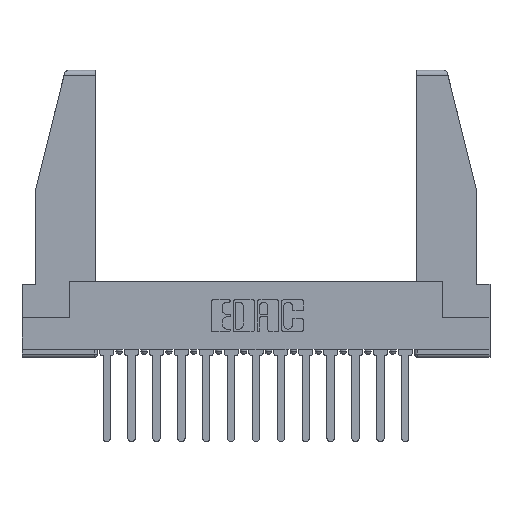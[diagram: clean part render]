
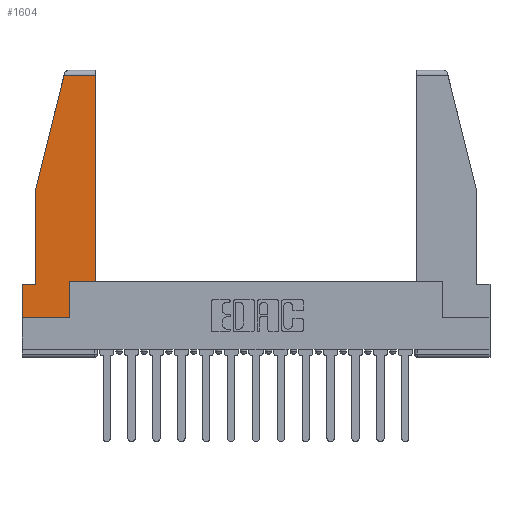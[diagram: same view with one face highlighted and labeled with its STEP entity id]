
A CAD part, top view. The second image highlights one B-rep face of the part: STEP entity #1604.
In plain terms, the highlighted planar face has unit normal (0, 0, 1).
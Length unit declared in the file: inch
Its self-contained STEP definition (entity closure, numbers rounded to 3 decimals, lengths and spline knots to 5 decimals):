
#199 = ORIENTED_EDGE ( 'NONE', *, *, #250, .T. ) ;
#250 = EDGE_CURVE ( 'NONE', #10235, #15832, #759, .T. ) ;
#589 = EDGE_LOOP ( 'NONE', ( #4565, #8580, #4721, #5813, #199, #5199, #11838, #7251, #9016 ) ) ;
#639 = AXIS2_PLACEMENT_3D ( 'NONE', #9587, #5339, #2652 ) ;
#759 = LINE ( 'NONE', #16954, #15724 ) ;
#966 = DIRECTION ( 'NONE',  ( -0.239, -0.971, 0. ) ) ;
#1041 = CARTESIAN_POINT ( 'NONE',  ( 0.461, 1.52, 0. ) ) ;
#1324 = CARTESIAN_POINT ( 'NONE',  ( 0.271, 1.55, 0. ) ) ;
#1604 = ADVANCED_FACE ( 'NONE', ( #13386 ), #8262, .T. ) ;
#1824 = VECTOR ( 'NONE', #15880, 39.37008 ) ;
#1844 = DIRECTION ( 'NONE',  ( 0., -1., 0. ) ) ;
#2352 = CARTESIAN_POINT ( 'NONE',  ( 0.461, 0.223, 0. ) ) ;
#2359 = LINE ( 'NONE', #17128, #13360 ) ;
#2652 = DIRECTION ( 'NONE',  ( 1., 0., 0. ) ) ;
#2764 = CARTESIAN_POINT ( 'NONE',  ( 0.086, 0.8, 0. ) ) ;
#3271 = DIRECTION ( 'NONE',  ( -1., 0., 0. ) ) ;
#3292 = EDGE_CURVE ( 'NONE', #16701, #4306, #10634, .T. ) ;
#3340 = EDGE_CURVE ( 'NONE', #10480, #16760, #6547, .T. ) ;
#3363 = CARTESIAN_POINT ( 'NONE',  ( 0.086, 0.21, 0. ) ) ;
#3607 = EDGE_CURVE ( 'NONE', #9724, #10235, #15353, .T. ) ;
#4048 = LINE ( 'NONE', #9469, #16231 ) ;
#4306 = VERTEX_POINT ( 'NONE', #5192 ) ;
#4406 = CARTESIAN_POINT ( 'NONE',  ( 0., 0.21, 0. ) ) ;
#4565 = ORIENTED_EDGE ( 'NONE', *, *, #11818, .T. ) ;
#4721 = ORIENTED_EDGE ( 'NONE', *, *, #7964, .T. ) ;
#5113 = EDGE_CURVE ( 'NONE', #16760, #8881, #4048, .T. ) ;
#5192 = CARTESIAN_POINT ( 'NONE',  ( 0.2636, 1.52, 0. ) ) ;
#5199 = ORIENTED_EDGE ( 'NONE', *, *, #11905, .T. ) ;
#5339 = DIRECTION ( 'NONE',  ( 0., 0., 1. ) ) ;
#5774 = CARTESIAN_POINT ( 'NONE',  ( 0.086, 0.8, 0. ) ) ;
#5813 = ORIENTED_EDGE ( 'NONE', *, *, #3607, .T. ) ;
#6547 = LINE ( 'NONE', #16063, #16580 ) ;
#6697 = DIRECTION ( 'NONE',  ( 1., 0., 0. ) ) ;
#6747 = VECTOR ( 'NONE', #966, 39.37008 ) ;
#6892 = DIRECTION ( 'NONE',  ( 0., -1., 0. ) ) ;
#7251 = ORIENTED_EDGE ( 'NONE', *, *, #3340, .T. ) ;
#7964 = EDGE_CURVE ( 'NONE', #4306, #9724, #10735, .T. ) ;
#8262 = PLANE ( 'NONE',  #639 ) ;
#8447 = CARTESIAN_POINT ( 'NONE',  ( 0.297, 0.223, 0. ) ) ;
#8580 = ORIENTED_EDGE ( 'NONE', *, *, #3292, .T. ) ;
#8881 = VERTEX_POINT ( 'NONE', #2352 ) ;
#9016 = ORIENTED_EDGE ( 'NONE', *, *, #5113, .T. ) ;
#9469 = CARTESIAN_POINT ( 'NONE',  ( 0.297, 0.223, 0. ) ) ;
#9559 = DIRECTION ( 'NONE',  ( 1., 0., 0. ) ) ;
#9587 = CARTESIAN_POINT ( 'NONE',  ( 0., 0., 0. ) ) ;
#9724 = VERTEX_POINT ( 'NONE', #2764 ) ;
#10235 = VERTEX_POINT ( 'NONE', #3363 ) ;
#10377 = CARTESIAN_POINT ( 'NONE',  ( 0., 1.52, 0. ) ) ;
#10480 = VERTEX_POINT ( 'NONE', #10869 ) ;
#10634 = LINE ( 'NONE', #10377, #1824 ) ;
#10735 = LINE ( 'NONE', #1324, #6747 ) ;
#10869 = CARTESIAN_POINT ( 'NONE',  ( 0.297, 0., 0. ) ) ;
#11037 = CARTESIAN_POINT ( 'NONE',  ( 0., 0., 0. ) ) ;
#11818 = EDGE_CURVE ( 'NONE', #8881, #16701, #2359, .T. ) ;
#11838 = ORIENTED_EDGE ( 'NONE', *, *, #12312, .T. ) ;
#11905 = EDGE_CURVE ( 'NONE', #15832, #15346, #13551, .T. ) ;
#12312 = EDGE_CURVE ( 'NONE', #15346, #10480, #16478, .T. ) ;
#12479 = CARTESIAN_POINT ( 'NONE',  ( 0., 0.21, 0. ) ) ;
#12815 = VECTOR ( 'NONE', #6892, 39.37008 ) ;
#13103 = VECTOR ( 'NONE', #6697, 39.37008 ) ;
#13360 = VECTOR ( 'NONE', #16051, 39.37008 ) ;
#13386 = FACE_OUTER_BOUND ( 'NONE', #589, .T. ) ;
#13551 = LINE ( 'NONE', #12479, #12815 ) ;
#15346 = VERTEX_POINT ( 'NONE', #16434 ) ;
#15353 = LINE ( 'NONE', #5774, #16675 ) ;
#15724 = VECTOR ( 'NONE', #3271, 39.37008 ) ;
#15798 = DIRECTION ( 'NONE',  ( 0., 1., 0. ) ) ;
#15832 = VERTEX_POINT ( 'NONE', #4406 ) ;
#15880 = DIRECTION ( 'NONE',  ( -1., 0., 0. ) ) ;
#16051 = DIRECTION ( 'NONE',  ( 0., 1., 0. ) ) ;
#16063 = CARTESIAN_POINT ( 'NONE',  ( 0.297, 0., 0. ) ) ;
#16231 = VECTOR ( 'NONE', #9559, 39.37008 ) ;
#16434 = CARTESIAN_POINT ( 'NONE',  ( 0., 0., 0. ) ) ;
#16478 = LINE ( 'NONE', #11037, #13103 ) ;
#16580 = VECTOR ( 'NONE', #15798, 39.37008 ) ;
#16675 = VECTOR ( 'NONE', #1844, 39.37008 ) ;
#16701 = VERTEX_POINT ( 'NONE', #1041 ) ;
#16760 = VERTEX_POINT ( 'NONE', #8447 ) ;
#16954 = CARTESIAN_POINT ( 'NONE',  ( 0., 0.21, 0. ) ) ;
#17128 = CARTESIAN_POINT ( 'NONE',  ( 0.461, 0.223, 0. ) ) ;
